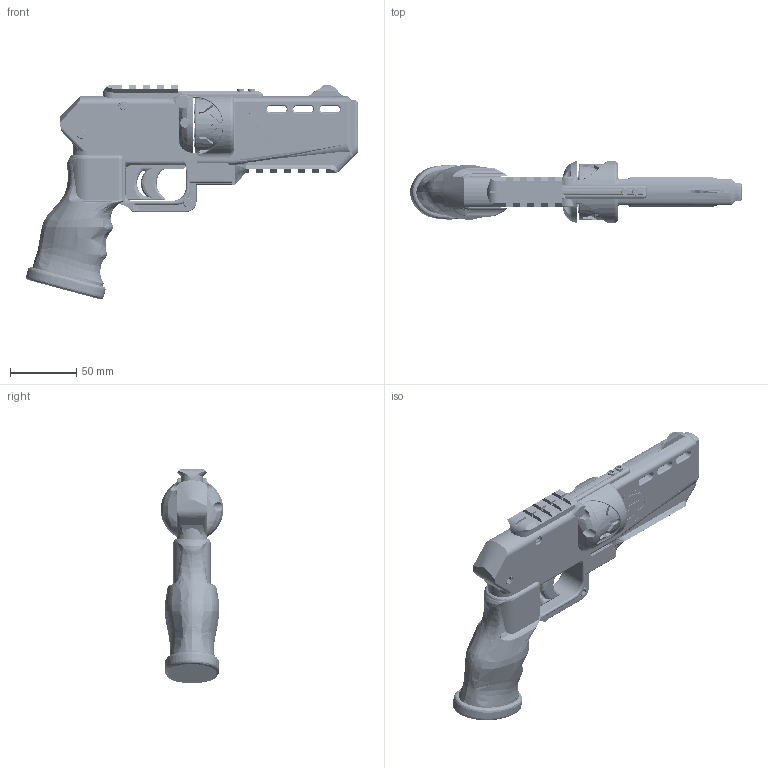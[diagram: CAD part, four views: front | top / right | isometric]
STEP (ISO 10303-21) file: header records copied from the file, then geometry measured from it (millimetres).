
FILE_DESCRIPTION(/* description */ (''),/* implementation_level */ '2;1');
FILE_NAME(/* name */ 'ImuraZip Final Working 22032020 wo.step',/* time_stamp */ '2020-03-22T19:45:51+01:00',/* author */ (''),/* organization */ (''),/* preprocessor_version */ 'ST-DEVELOPER v18',/* originating_system */ 'Autodesk Translation Framework v8.12.0.6',/* authorisation */ '');
FILE_SCHEMA (('AUTOMOTIVE_DESIGN { 1 0 10303 214 3 1 1 }'));
Products named in the file (60): (Unsaved); ImuraZip; FrameParts; ImuraBarrel; Imura_V2_Cylinder; 22LR; Cylinder Rod 8mm; Cylinder; Chamber Inserts; Inserts 25mm x 5; Barrel Front; Locking Lever; Barrel; FramePin 23x5mm; Component53; Rail; RailPin; Rail (1); Frame; Half Right ; Right Frame; Cover Right; Release Pin 8mm; Component52; Half Left 1 Spring; Left Frame; Cover Left; Internals; ImuraTrigger; SpringTrigger 1 (1); SpringTrigger 2 (1); Trigger ; Trigger (1); ImuraSearV4; Sear; Pin (1); ImuraStriker; Firing Pin; Sriker; Spring (1) ...
Assembly tree (59 placements, depth 7):
  (Unsaved)
    ImuraZip
      FrameParts
        ImuraBarrel
          Imura_V2_Cylinder
            22LR
            Cylinder Rod 8mm
            Cylinder
            Chamber Inserts
              Inserts 25mm x 5
          Barrel Front
          Locking Lever
          Barrel
          FramePin 23x5mm
            Component53
        Rail
          RailPin
          Rail (1)
        Frame
          Half Right 
            Right Frame
            Cover Right
          Release Pin 8mm
            Component52
          Half Left 1 Spring
            Left Frame
            Cover Left
        Internals
          ImuraTrigger
            SpringTrigger 1 (1)
            SpringTrigger 2 (1)
            Trigger 
              Trigger (1)
          ImuraSearV4
            Sear
            Pin (1)
          ImuraStriker
            Firing Pin
            Sriker
            Spring (1)
          ImuraFlapper
            FlapperSpring
            FlapperV4
            Pin
      Grip
        grip_1
        Bottom Plug
      Screws
        M3 x 14mm
        M4 x 16mm
        M4 x 16mm 2
        M4 x 16mm 3
        M3 x 14mm 2
        M3 x 14mm 2 3
        M3 x 10mm
        M3 x 10mm 2
      Ball Bearings
        Bearing 8x16x5mm 
        Bearing 8x16x5mm  2
        Bearing 8x16x5mm  3
Bounding box: 250.11 x 47 x 161.7 mm (x, y, z)
Volume: 383494.5 mm3; surface area: 170363 mm2
Topology: 53 solids, 63 shells, 2771 faces, 7885 edges, 5351 vertices
Faces by surface type: cylinder 963, plane 892, bspline 741, torus 104, cone 39, sphere 32
Full cylindrical faces by diameter (mm): 0.793 x8, 1.5 x3, 2 x2, 2.356 x119, 2.529 x81, 3.086 x85, 3.25 x2, 3.3 x3, 3.332 x48, 3.5 x1, 4 x9, 4.109 x28, 4.11 x14, 4.2 x2, 4.25 x2, 4.5 x4, 4.7 x1, 4.8 x4, 5 x10, 5.1 x2, 5.3 x1, 5.4 x5, 5.5 x10, 5.588 x32, 5.69 x8, 5.715 x24, 6 x13, 6.9 x3, 7.1 x4, 7.2 x1
Entity records: 340211 total; most frequent: CARTESIAN_POINT 272511, ORIENTED_EDGE 15704, DIRECTION 10851, EDGE_CURVE 7852, VERTEX_POINT 5350, AXIS2_PLACEMENT_3D 3847, LINE 3157, VECTOR 3157
